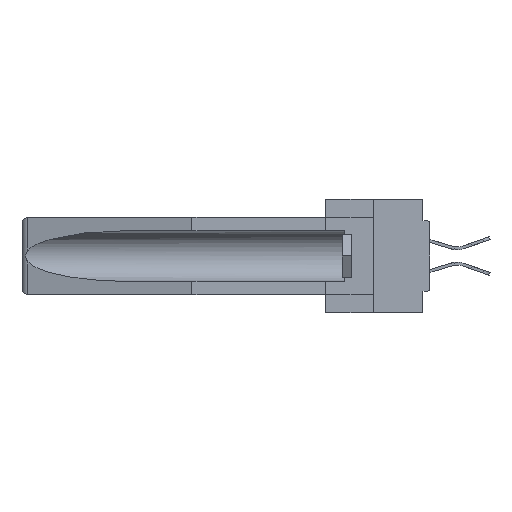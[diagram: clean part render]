
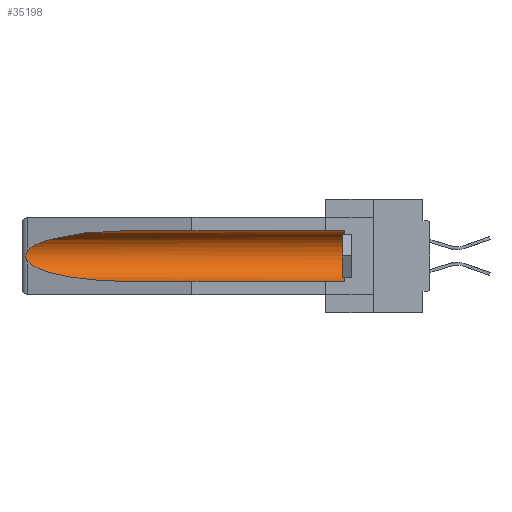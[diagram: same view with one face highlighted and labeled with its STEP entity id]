
A CAD part, left-side view. The second image highlights one B-rep face of the part: STEP entity #35198.
In plain terms, the highlighted cylindrical face has radius 2.857 mm (diameter 5.715 mm), a partial arc.
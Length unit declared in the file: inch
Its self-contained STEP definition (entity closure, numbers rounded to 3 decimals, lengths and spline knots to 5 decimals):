
#651 = CARTESIAN_POINT ( 'NONE',  ( 0.2673, 1.53269, -0.17917 ) ) ;
#658 = DIRECTION ( 'NONE',  ( 0., -1., 0. ) ) ;
#903 =( BOUNDED_CURVE ( )  B_SPLINE_CURVE ( 3, ( #21025, #31505, #24332, #2684 ),
 .UNSPECIFIED., .F., .T. ) 
 B_SPLINE_CURVE_WITH_KNOTS ( ( 4, 4 ),
 ( 4.71239, 6.08839 ),
 .UNSPECIFIED. ) 
 CURVE ( )  GEOMETRIC_REPRESENTATION_ITEM ( )  RATIONAL_B_SPLINE_CURVE ( ( 1., 0.848, 0.848, 1. ) ) 
 REPRESENTATION_ITEM ( '' )  );
#1273 = CIRCLE ( 'NONE', #2891, 0.1125 ) ;
#2684 = CARTESIAN_POINT ( 'NONE',  ( 0.26537, 1.52718, -0.14972 ) ) ;
#2891 = AXIS2_PLACEMENT_3D ( 'NONE', #36420, #658, #18042 ) ;
#3617 = CARTESIAN_POINT ( 'NONE',  ( 0.155, -0.30754, -0.059 ) ) ;
#4098 = EDGE_CURVE ( 'NONE', #41578, #31437, #8862, .T. ) ;
#4314 = CARTESIAN_POINT ( 'NONE',  ( 0.26537, 1.52718, -0.19328 ) ) ;
#4825 = EDGE_LOOP ( 'NONE', ( #33100, #6074, #22554, #28853, #25674, #40105 ) ) ;
#6074 = ORIENTED_EDGE ( 'NONE', *, *, #18942, .T. ) ;
#7465 = CARTESIAN_POINT ( 'NONE',  ( 0.26537, 1.52718, -0.14972 ) ) ;
#7911 = DIRECTION ( 'NONE',  ( 0., 1., 0. ) ) ;
#7945 = CARTESIAN_POINT ( 'NONE',  ( 0.2675, 1.53308, -0.17534 ) ) ;
#8862 = LINE ( 'NONE', #3617, #18476 ) ;
#11449 = EDGE_CURVE ( 'NONE', #11894, #41578, #1273, .T. ) ;
#11894 = VERTEX_POINT ( 'NONE', #25712 ) ;
#12456 = CARTESIAN_POINT ( 'NONE',  ( 0.155, -0.30754, -0.1715 ) ) ;
#13241 = AXIS2_PLACEMENT_3D ( 'NONE', #12456, #29902, #44629 ) ;
#15061 = CARTESIAN_POINT ( 'NONE',  ( 0.21114, 1.30732, -0.284 ) ) ;
#15208 = DIRECTION ( 'NONE',  ( 0., 1., 0. ) ) ;
#17691 = B_SPLINE_CURVE_WITH_KNOTS ( 'NONE', 3,
 ( #7465, #36567, #18202, #40181, #36255, #7945, #651, #39855, #21833, #43441 ),
 .UNSPECIFIED., .F., .F.,
 ( 4, 2, 2, 2, 4 ),
 ( 0., 0.00029, 0.00058, 0.00087, 0.00117 ),
 .UNSPECIFIED. ) ;
#18042 = DIRECTION ( 'NONE',  ( 0., 0., 1. ) ) ;
#18202 = CARTESIAN_POINT ( 'NONE',  ( 0.26654, 1.53092, -0.15636 ) ) ;
#18476 = VECTOR ( 'NONE', #7911, 39.37008 ) ;
#18544 = CARTESIAN_POINT ( 'NONE',  ( 0.25451, 1.48313, -0.24835 ) ) ;
#18942 = EDGE_CURVE ( 'NONE', #39068, #42992, #17691, .T. ) ;
#20730 = CARTESIAN_POINT ( 'NONE',  ( 0.155, 1.07973, -0.284 ) ) ;
#20809 = CYLINDRICAL_SURFACE ( 'NONE', #13241, 0.1125 ) ;
#20904 = VECTOR ( 'NONE', #15208, 39.37008 ) ;
#21025 = CARTESIAN_POINT ( 'NONE',  ( 0.155, 1.07973, -0.059 ) ) ;
#21833 = CARTESIAN_POINT ( 'NONE',  ( 0.26597, 1.5296, -0.19026 ) ) ;
#22554 = ORIENTED_EDGE ( 'NONE', *, *, #27971, .T. ) ;
#23091 = VERTEX_POINT ( 'NONE', #20730 ) ;
#24332 = CARTESIAN_POINT ( 'NONE',  ( 0.25451, 1.48313, -0.09465 ) ) ;
#25674 = ORIENTED_EDGE ( 'NONE', *, *, #11449, .T. ) ;
#25712 = CARTESIAN_POINT ( 'NONE',  ( 0.155, 0.126, -0.284 ) ) ;
#27008 = CARTESIAN_POINT ( 'NONE',  ( 0.26537, 1.52718, -0.14972 ) ) ;
#27971 = EDGE_CURVE ( 'NONE', #42992, #23091, #30367, .T. ) ;
#28853 = ORIENTED_EDGE ( 'NONE', *, *, #34308, .F. ) ;
#29132 = CARTESIAN_POINT ( 'NONE',  ( 0.155, 1.07973, -0.059 ) ) ;
#29902 = DIRECTION ( 'NONE',  ( 0., 1., 0. ) ) ;
#30367 =( BOUNDED_CURVE ( )  B_SPLINE_CURVE ( 3, ( #4314, #18544, #15061, #33096 ),
 .UNSPECIFIED., .F., .F. ) 
 B_SPLINE_CURVE_WITH_KNOTS ( ( 4, 4 ),
 ( 0.1948, 1.5708 ),
 .UNSPECIFIED. ) 
 CURVE ( )  GEOMETRIC_REPRESENTATION_ITEM ( )  RATIONAL_B_SPLINE_CURVE ( ( 1., 0.848, 0.848, 1. ) ) 
 REPRESENTATION_ITEM ( '' )  );
#31437 = VERTEX_POINT ( 'NONE', #29132 ) ;
#31505 = CARTESIAN_POINT ( 'NONE',  ( 0.21114, 1.30732, -0.059 ) ) ;
#32891 = CARTESIAN_POINT ( 'NONE',  ( 0.155, 0.126, -0.059 ) ) ;
#33096 = CARTESIAN_POINT ( 'NONE',  ( 0.155, 1.07973, -0.284 ) ) ;
#33100 = ORIENTED_EDGE ( 'NONE', *, *, #45509, .T. ) ;
#34308 = EDGE_CURVE ( 'NONE', #11894, #23091, #46647, .T. ) ;
#35198 = ADVANCED_FACE ( 'NONE', ( #44398 ), #20809, .F. ) ;
#36255 = CARTESIAN_POINT ( 'NONE',  ( 0.2675, 1.53308, -0.16763 ) ) ;
#36420 = CARTESIAN_POINT ( 'NONE',  ( 0.155, 0.126, -0.1715 ) ) ;
#36567 = CARTESIAN_POINT ( 'NONE',  ( 0.26597, 1.52961, -0.15275 ) ) ;
#39068 = VERTEX_POINT ( 'NONE', #27008 ) ;
#39855 = CARTESIAN_POINT ( 'NONE',  ( 0.26655, 1.53094, -0.18657 ) ) ;
#40105 = ORIENTED_EDGE ( 'NONE', *, *, #4098, .T. ) ;
#40181 = CARTESIAN_POINT ( 'NONE',  ( 0.2673, 1.5327, -0.16383 ) ) ;
#40327 = CARTESIAN_POINT ( 'NONE',  ( 0.155, -0.30754, -0.284 ) ) ;
#41578 = VERTEX_POINT ( 'NONE', #32891 ) ;
#41884 = CARTESIAN_POINT ( 'NONE',  ( 0.26537, 1.52718, -0.19328 ) ) ;
#42992 = VERTEX_POINT ( 'NONE', #41884 ) ;
#43441 = CARTESIAN_POINT ( 'NONE',  ( 0.26537, 1.52718, -0.19328 ) ) ;
#44398 = FACE_OUTER_BOUND ( 'NONE', #4825, .T. ) ;
#44629 = DIRECTION ( 'NONE',  ( 0., 0., 1. ) ) ;
#45509 = EDGE_CURVE ( 'NONE', #31437, #39068, #903, .T. ) ;
#46647 = LINE ( 'NONE', #40327, #20904 ) ;
